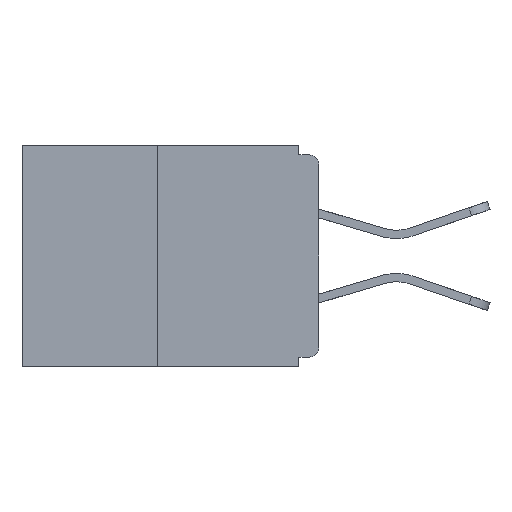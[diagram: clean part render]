
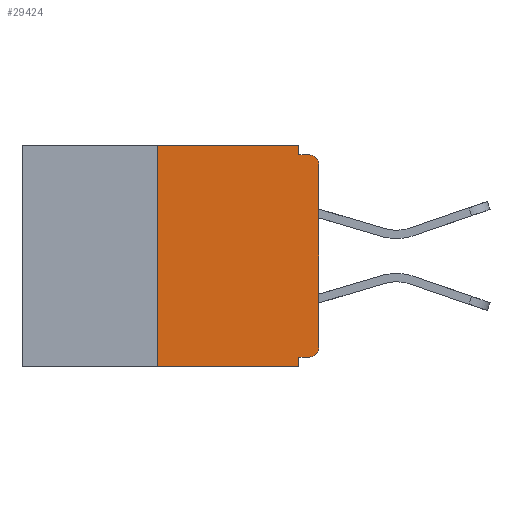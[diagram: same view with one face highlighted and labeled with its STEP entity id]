
A CAD part, left-side view. The second image highlights one B-rep face of the part: STEP entity #29424.
In plain terms, the highlighted planar face has unit normal (-1, 0, 0).
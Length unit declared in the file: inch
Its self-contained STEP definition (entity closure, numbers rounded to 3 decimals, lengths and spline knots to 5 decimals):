
#681 = EDGE_CURVE ( 'NONE', #6401, #25196, #4682, .T. ) ;
#827 = CARTESIAN_POINT ( 'NONE',  ( 0., 0., -0.313 ) ) ;
#1055 = EDGE_LOOP ( 'NONE', ( #3811, #27706, #27921, #19504, #20133, #23958, #28793, #13270, #16362, #5691 ) ) ;
#1234 = DIRECTION ( 'NONE',  ( 1., 0., 0. ) ) ;
#1350 = EDGE_CURVE ( 'NONE', #3975, #3213, #5781, .T. ) ;
#1394 = EDGE_CURVE ( 'NONE', #26369, #24748, #20902, .T. ) ;
#1797 = VERTEX_POINT ( 'NONE', #22036 ) ;
#1911 = LINE ( 'NONE', #25922, #12433 ) ;
#2748 = EDGE_CURVE ( 'NONE', #27347, #6754, #1911, .T. ) ;
#2943 = PLANE ( 'NONE',  #10463 ) ;
#3213 = VERTEX_POINT ( 'NONE', #28748 ) ;
#3580 = VECTOR ( 'NONE', #8572, 39.37008 ) ;
#3811 = ORIENTED_EDGE ( 'NONE', *, *, #11718, .F. ) ;
#3975 = VERTEX_POINT ( 'NONE', #6642 ) ;
#4476 = VECTOR ( 'NONE', #25434, 39.37008 ) ;
#4682 = LINE ( 'NONE', #14038, #9366 ) ;
#5060 = CARTESIAN_POINT ( 'NONE',  ( 0., 0., -0.03 ) ) ;
#5263 = DIRECTION ( 'NONE',  ( 0., 0., -1. ) ) ;
#5691 = ORIENTED_EDGE ( 'NONE', *, *, #28385, .F. ) ;
#5781 = LINE ( 'NONE', #29427, #3580 ) ;
#5846 = AXIS2_PLACEMENT_3D ( 'NONE', #11640, #14235, #25826 ) ;
#6025 = CARTESIAN_POINT ( 'NONE',  ( 0., 0.015, -0.313 ) ) ;
#6401 = VERTEX_POINT ( 'NONE', #827 ) ;
#6465 = LINE ( 'NONE', #12746, #11519 ) ;
#6532 = AXIS2_PLACEMENT_3D ( 'NONE', #6025, #12889, #26950 ) ;
#6565 = DIRECTION ( 'NONE',  ( 0., 0., 1. ) ) ;
#6642 = CARTESIAN_POINT ( 'NONE',  ( 0., 0.031, -0.015 ) ) ;
#6754 = VERTEX_POINT ( 'NONE', #12364 ) ;
#6918 = CARTESIAN_POINT ( 'NONE',  ( 0., 0.031, -0.343 ) ) ;
#8557 = CARTESIAN_POINT ( 'NONE',  ( 0., 0.031, -0.328 ) ) ;
#8572 = DIRECTION ( 'NONE',  ( 0., -1., 0. ) ) ;
#8952 = CIRCLE ( 'NONE', #6532, 0.015 ) ;
#9366 = VECTOR ( 'NONE', #9628, 39.37008 ) ;
#9628 = DIRECTION ( 'NONE',  ( 0., 0., 1. ) ) ;
#9691 = DIRECTION ( 'NONE',  ( 0., 0., -1. ) ) ;
#10286 = CARTESIAN_POINT ( 'NONE',  ( 0., 0.25, -0.343 ) ) ;
#10463 = AXIS2_PLACEMENT_3D ( 'NONE', #23592, #1234, #5263 ) ;
#11403 = LINE ( 'NONE', #20385, #18930 ) ;
#11519 = VECTOR ( 'NONE', #12658, 39.37008 ) ;
#11640 = CARTESIAN_POINT ( 'NONE',  ( 0., 0.015, -0.03 ) ) ;
#11718 = EDGE_CURVE ( 'NONE', #23513, #1797, #6465, .T. ) ;
#12358 = EDGE_CURVE ( 'NONE', #26369, #6401, #8952, .T. ) ;
#12364 = CARTESIAN_POINT ( 'NONE',  ( 0., 0.031, -0.343 ) ) ;
#12433 = VECTOR ( 'NONE', #16662, 39.37008 ) ;
#12658 = DIRECTION ( 'NONE',  ( 0., -1., 0. ) ) ;
#12746 = CARTESIAN_POINT ( 'NONE',  ( 0., 0.46, 0. ) ) ;
#12801 = LINE ( 'NONE', #6918, #4476 ) ;
#12889 = DIRECTION ( 'NONE',  ( -1., 0., 0. ) ) ;
#13270 = ORIENTED_EDGE ( 'NONE', *, *, #29304, .T. ) ;
#13369 = CIRCLE ( 'NONE', #5846, 0.015 ) ;
#14038 = CARTESIAN_POINT ( 'NONE',  ( 0., 0., 0. ) ) ;
#14235 = DIRECTION ( 'NONE',  ( -1., 0., 0. ) ) ;
#14310 = CARTESIAN_POINT ( 'NONE',  ( 0., 0.031, 0. ) ) ;
#16217 = VECTOR ( 'NONE', #9691, 39.37008 ) ;
#16362 = ORIENTED_EDGE ( 'NONE', *, *, #1350, .F. ) ;
#16587 = FACE_OUTER_BOUND ( 'NONE', #1055, .T. ) ;
#16662 = DIRECTION ( 'NONE',  ( 0., -1., 0. ) ) ;
#17190 = EDGE_CURVE ( 'NONE', #24748, #6754, #12801, .T. ) ;
#18930 = VECTOR ( 'NONE', #6565, 39.37008 ) ;
#19504 = ORIENTED_EDGE ( 'NONE', *, *, #17190, .F. ) ;
#20133 = ORIENTED_EDGE ( 'NONE', *, *, #1394, .F. ) ;
#20385 = CARTESIAN_POINT ( 'NONE',  ( 0., 0.25, 0. ) ) ;
#20387 = EDGE_CURVE ( 'NONE', #27347, #23513, #11403, .T. ) ;
#20902 = LINE ( 'NONE', #29724, #25644 ) ;
#22036 = CARTESIAN_POINT ( 'NONE',  ( 0., 0.031, 0. ) ) ;
#22441 = LINE ( 'NONE', #14310, #16217 ) ;
#23360 = CARTESIAN_POINT ( 'NONE',  ( 0., 0.25, 0. ) ) ;
#23513 = VERTEX_POINT ( 'NONE', #23360 ) ;
#23592 = CARTESIAN_POINT ( 'NONE',  ( 0., 0.46, 0. ) ) ;
#23958 = ORIENTED_EDGE ( 'NONE', *, *, #12358, .T. ) ;
#24748 = VERTEX_POINT ( 'NONE', #8557 ) ;
#24752 = DIRECTION ( 'NONE',  ( 0., 1., 0. ) ) ;
#25196 = VERTEX_POINT ( 'NONE', #5060 ) ;
#25434 = DIRECTION ( 'NONE',  ( 0., 0., -1. ) ) ;
#25644 = VECTOR ( 'NONE', #24752, 39.37008 ) ;
#25826 = DIRECTION ( 'NONE',  ( 0., 0., -1. ) ) ;
#25922 = CARTESIAN_POINT ( 'NONE',  ( 0., 0.46, -0.343 ) ) ;
#26369 = VERTEX_POINT ( 'NONE', #27988 ) ;
#26950 = DIRECTION ( 'NONE',  ( 0., 0., -1. ) ) ;
#27347 = VERTEX_POINT ( 'NONE', #10286 ) ;
#27706 = ORIENTED_EDGE ( 'NONE', *, *, #20387, .F. ) ;
#27921 = ORIENTED_EDGE ( 'NONE', *, *, #2748, .T. ) ;
#27988 = CARTESIAN_POINT ( 'NONE',  ( 0., 0.015, -0.328 ) ) ;
#28385 = EDGE_CURVE ( 'NONE', #1797, #3975, #22441, .T. ) ;
#28748 = CARTESIAN_POINT ( 'NONE',  ( 0., 0.015, -0.015 ) ) ;
#28793 = ORIENTED_EDGE ( 'NONE', *, *, #681, .T. ) ;
#29304 = EDGE_CURVE ( 'NONE', #25196, #3213, #13369, .T. ) ;
#29424 = ADVANCED_FACE ( 'NONE', ( #16587 ), #2943, .F. ) ;
#29427 = CARTESIAN_POINT ( 'NONE',  ( 0., 0., -0.015 ) ) ;
#29724 = CARTESIAN_POINT ( 'NONE',  ( 0., 0., -0.328 ) ) ;
